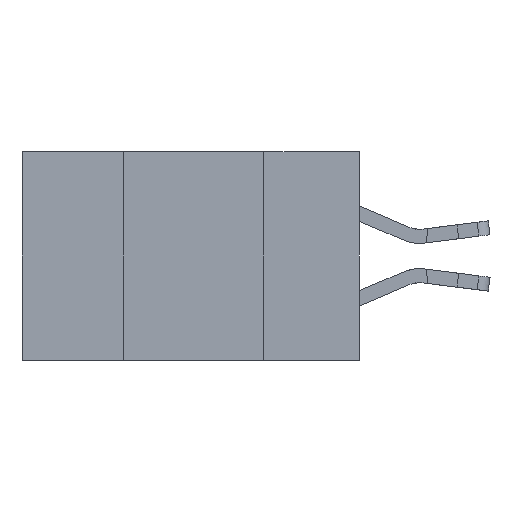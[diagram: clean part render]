
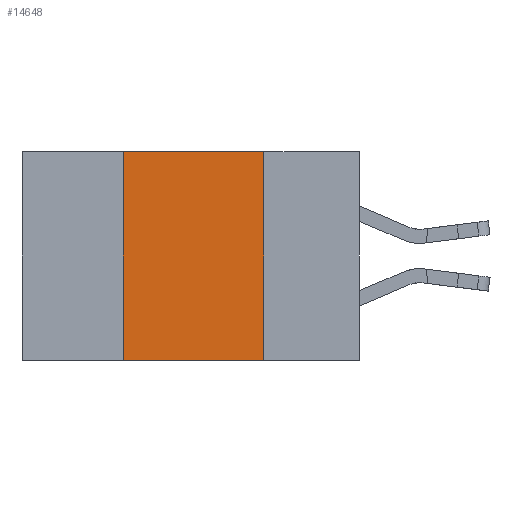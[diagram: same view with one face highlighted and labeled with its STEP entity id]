
A CAD part, left-side view. The second image highlights one B-rep face of the part: STEP entity #14648.
In plain terms, the highlighted planar face has unit normal (-1, 0, 0).
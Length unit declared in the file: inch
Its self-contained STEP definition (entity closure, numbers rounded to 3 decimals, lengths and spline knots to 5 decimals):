
#4 = VECTOR ( 'NONE', #15558, 39.37008 ) ;
#476 = LINE ( 'NONE', #11190, #4 ) ;
#583 = CARTESIAN_POINT ( 'NONE',  ( 0., 0.6, -0.37 ) ) ;
#2533 = VECTOR ( 'NONE', #3746, 39.37008 ) ;
#2544 = VERTEX_POINT ( 'NONE', #13775 ) ;
#3491 = EDGE_CURVE ( 'NONE', #7810, #12341, #476, .T. ) ;
#3746 = DIRECTION ( 'NONE',  ( 0., 0., 1. ) ) ;
#4274 = VECTOR ( 'NONE', #9812, 39.37008 ) ;
#4999 = VECTOR ( 'NONE', #13941, 39.37008 ) ;
#7001 = AXIS2_PLACEMENT_3D ( 'NONE', #17383, #8667, #18856 ) ;
#7810 = VERTEX_POINT ( 'NONE', #12008 ) ;
#8667 = DIRECTION ( 'NONE',  ( 1., 0., 0. ) ) ;
#9772 = EDGE_CURVE ( 'NONE', #2544, #7810, #17309, .T. ) ;
#9812 = DIRECTION ( 'NONE',  ( 0., 0., -1. ) ) ;
#10465 = ORIENTED_EDGE ( 'NONE', *, *, #18499, .F. ) ;
#10937 = ORIENTED_EDGE ( 'NONE', *, *, #9772, .F. ) ;
#11190 = CARTESIAN_POINT ( 'NONE',  ( 0., 0.6, 0. ) ) ;
#11664 = EDGE_LOOP ( 'NONE', ( #10465, #14371, #10937, #18623 ) ) ;
#12008 = CARTESIAN_POINT ( 'NONE',  ( 0., 0.42, 0. ) ) ;
#12341 = VERTEX_POINT ( 'NONE', #15037 ) ;
#12726 = CARTESIAN_POINT ( 'NONE',  ( 0., 0.42, 0. ) ) ;
#13051 = PLANE ( 'NONE',  #7001 ) ;
#13775 = CARTESIAN_POINT ( 'NONE',  ( 0., 0.42, -0.37 ) ) ;
#13941 = DIRECTION ( 'NONE',  ( 0., -1., 0. ) ) ;
#14178 = CARTESIAN_POINT ( 'NONE',  ( 0., 0.17, -0.37 ) ) ;
#14371 = ORIENTED_EDGE ( 'NONE', *, *, #3491, .F. ) ;
#14648 = ADVANCED_FACE ( 'NONE', ( #18826 ), #13051, .F. ) ;
#15018 = EDGE_CURVE ( 'NONE', #2544, #16602, #16311, .T. ) ;
#15037 = CARTESIAN_POINT ( 'NONE',  ( 0., 0.17, 0. ) ) ;
#15187 = LINE ( 'NONE', #17072, #4274 ) ;
#15558 = DIRECTION ( 'NONE',  ( 0., -1., 0. ) ) ;
#16311 = LINE ( 'NONE', #583, #4999 ) ;
#16602 = VERTEX_POINT ( 'NONE', #14178 ) ;
#17072 = CARTESIAN_POINT ( 'NONE',  ( 0., 0.17, 0. ) ) ;
#17309 = LINE ( 'NONE', #12726, #2533 ) ;
#17383 = CARTESIAN_POINT ( 'NONE',  ( 0., 0.6, 0. ) ) ;
#18499 = EDGE_CURVE ( 'NONE', #12341, #16602, #15187, .T. ) ;
#18623 = ORIENTED_EDGE ( 'NONE', *, *, #15018, .T. ) ;
#18826 = FACE_OUTER_BOUND ( 'NONE', #11664, .T. ) ;
#18856 = DIRECTION ( 'NONE',  ( 0., 0., -1. ) ) ;
